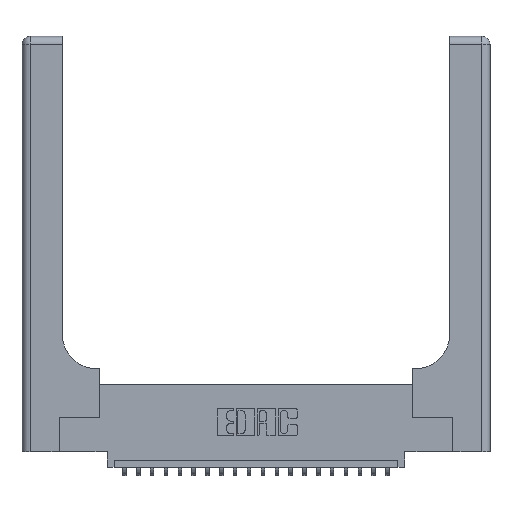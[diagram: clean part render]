
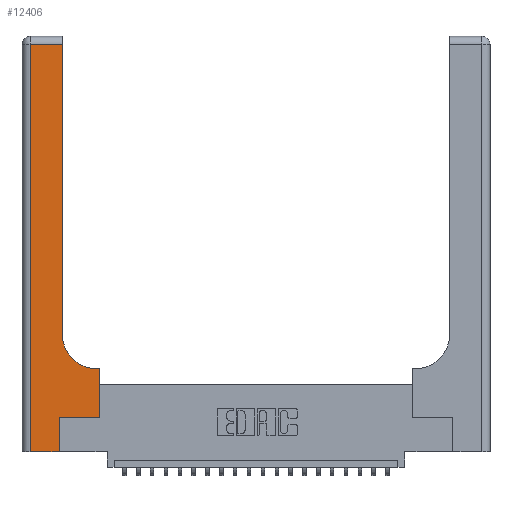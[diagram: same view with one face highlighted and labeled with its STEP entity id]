
A CAD part, top view. The second image highlights one B-rep face of the part: STEP entity #12406.
In plain terms, the highlighted planar face has unit normal (0, 0, 1).
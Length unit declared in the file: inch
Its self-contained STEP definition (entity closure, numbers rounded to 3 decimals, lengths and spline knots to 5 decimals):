
#960 = VECTOR ( 'NONE', #11926, 39.37008 ) ;
#1051 = LINE ( 'NONE', #10312, #22240 ) ;
#1221 = CARTESIAN_POINT ( 'NONE',  ( 0.2915, 0.6, 0.37 ) ) ;
#1324 = DIRECTION ( 'NONE',  ( -1., 0., 0. ) ) ;
#1668 = EDGE_CURVE ( 'NONE', #20339, #4295, #11186, .T. ) ;
#1721 = VERTEX_POINT ( 'NONE', #21738 ) ;
#1817 = CARTESIAN_POINT ( 'NONE',  ( 0.5585, 0.6, 0.37 ) ) ;
#2383 = ORIENTED_EDGE ( 'NONE', *, *, #4557, .T. ) ;
#3017 = VERTEX_POINT ( 'NONE', #7567 ) ;
#3099 = CARTESIAN_POINT ( 'NONE',  ( 0.269, 0., 0.37 ) ) ;
#3658 = EDGE_CURVE ( 'NONE', #6138, #20339, #19414, .T. ) ;
#3685 = ORIENTED_EDGE ( 'NONE', *, *, #5628, .T. ) ;
#3878 = VECTOR ( 'NONE', #6095, 39.37008 ) ;
#4277 = CARTESIAN_POINT ( 'NONE',  ( 0.06, 3., 0.37 ) ) ;
#4295 = VERTEX_POINT ( 'NONE', #11991 ) ;
#4314 = FACE_OUTER_BOUND ( 'NONE', #8168, .T. ) ;
#4333 = DIRECTION ( 'NONE',  ( -1., 0., 0. ) ) ;
#4454 = VECTOR ( 'NONE', #4813, 39.37008 ) ;
#4557 = EDGE_CURVE ( 'NONE', #19125, #6138, #18001, .T. ) ;
#4813 = DIRECTION ( 'NONE',  ( -1., 0., 0. ) ) ;
#5012 = VECTOR ( 'NONE', #18458, 39.37008 ) ;
#5111 = CARTESIAN_POINT ( 'NONE',  ( 0.06, 0., 0.37 ) ) ;
#5488 = CARTESIAN_POINT ( 'NONE',  ( 0.5585, 0.25, 0.37 ) ) ;
#5628 = EDGE_CURVE ( 'NONE', #4295, #3017, #12844, .T. ) ;
#5804 = EDGE_CURVE ( 'NONE', #1721, #12709, #6657, .T. ) ;
#6095 = DIRECTION ( 'NONE',  ( 0., -1., 0. ) ) ;
#6138 = VERTEX_POINT ( 'NONE', #5111 ) ;
#6259 = ORIENTED_EDGE ( 'NONE', *, *, #1668, .T. ) ;
#6657 = LINE ( 'NONE', #9618, #21048 ) ;
#6861 = ORIENTED_EDGE ( 'NONE', *, *, #21499, .T. ) ;
#7369 = VECTOR ( 'NONE', #10957, 39.37008 ) ;
#7567 = CARTESIAN_POINT ( 'NONE',  ( 0.5585, 0.25, 0.37 ) ) ;
#8168 = EDGE_LOOP ( 'NONE', ( #9216, #20726, #2383, #13592, #6259, #3685, #11124, #6861, #22693 ) ) ;
#8589 = DIRECTION ( 'NONE',  ( 1., 0., 0. ) ) ;
#8967 = CARTESIAN_POINT ( 'NONE',  ( 0.5415, 0.6, 0.37 ) ) ;
#9216 = ORIENTED_EDGE ( 'NONE', *, *, #5804, .T. ) ;
#9290 = AXIS2_PLACEMENT_3D ( 'NONE', #13443, #15250, #9794 ) ;
#9618 = CARTESIAN_POINT ( 'NONE',  ( 0.2915, 3., 0.37 ) ) ;
#9794 = DIRECTION ( 'NONE',  ( 1., 0., 0. ) ) ;
#10312 = CARTESIAN_POINT ( 'NONE',  ( 0., 2.94, 0.37 ) ) ;
#10370 = CARTESIAN_POINT ( 'NONE',  ( 0., 3., 0.37 ) ) ;
#10957 = DIRECTION ( 'NONE',  ( 0., 1., 0. ) ) ;
#11124 = ORIENTED_EDGE ( 'NONE', *, *, #13130, .T. ) ;
#11186 = LINE ( 'NONE', #3099, #960 ) ;
#11926 = DIRECTION ( 'NONE',  ( 0., 1., 0. ) ) ;
#11991 = CARTESIAN_POINT ( 'NONE',  ( 0.269, 0.25, 0.37 ) ) ;
#12149 = LINE ( 'NONE', #5488, #7369 ) ;
#12406 = ADVANCED_FACE ( 'NONE', ( #4314 ), #20334, .F. ) ;
#12709 = VERTEX_POINT ( 'NONE', #20183 ) ;
#12844 = LINE ( 'NONE', #17320, #14818 ) ;
#12972 = CARTESIAN_POINT ( 'NONE',  ( 0., 0., 0.37 ) ) ;
#13087 = CIRCLE ( 'NONE', #9290, 0.25 ) ;
#13130 = EDGE_CURVE ( 'NONE', #3017, #19410, #12149, .T. ) ;
#13443 = CARTESIAN_POINT ( 'NONE',  ( 0.5415, 0.85, 0.37 ) ) ;
#13592 = ORIENTED_EDGE ( 'NONE', *, *, #3658, .T. ) ;
#14125 = VERTEX_POINT ( 'NONE', #8967 ) ;
#14818 = VECTOR ( 'NONE', #8589, 39.37008 ) ;
#15250 = DIRECTION ( 'NONE',  ( 0., 0., -1. ) ) ;
#15996 = LINE ( 'NONE', #1221, #4454 ) ;
#17025 = CARTESIAN_POINT ( 'NONE',  ( 0.269, 0., 0.37 ) ) ;
#17320 = CARTESIAN_POINT ( 'NONE',  ( 0.269, 0.25, 0.37 ) ) ;
#18001 = LINE ( 'NONE', #4277, #3878 ) ;
#18458 = DIRECTION ( 'NONE',  ( 1., 0., 0. ) ) ;
#18508 = CARTESIAN_POINT ( 'NONE',  ( 0.06, 2.94, 0.37 ) ) ;
#19103 = DIRECTION ( 'NONE',  ( 0., 0., -1. ) ) ;
#19125 = VERTEX_POINT ( 'NONE', #18508 ) ;
#19410 = VERTEX_POINT ( 'NONE', #1817 ) ;
#19414 = LINE ( 'NONE', #12972, #5012 ) ;
#20173 = DIRECTION ( 'NONE',  ( 0., 1., 0. ) ) ;
#20183 = CARTESIAN_POINT ( 'NONE',  ( 0.2915, 2.94, 0.37 ) ) ;
#20334 = PLANE ( 'NONE',  #21235 ) ;
#20339 = VERTEX_POINT ( 'NONE', #17025 ) ;
#20726 = ORIENTED_EDGE ( 'NONE', *, *, #20926, .T. ) ;
#20926 = EDGE_CURVE ( 'NONE', #12709, #19125, #1051, .T. ) ;
#21048 = VECTOR ( 'NONE', #20173, 39.37008 ) ;
#21235 = AXIS2_PLACEMENT_3D ( 'NONE', #10370, #19103, #4333 ) ;
#21499 = EDGE_CURVE ( 'NONE', #19410, #14125, #15996, .T. ) ;
#21738 = CARTESIAN_POINT ( 'NONE',  ( 0.2915, 0.85, 0.37 ) ) ;
#22240 = VECTOR ( 'NONE', #1324, 39.37008 ) ;
#22693 = ORIENTED_EDGE ( 'NONE', *, *, #22932, .T. ) ;
#22932 = EDGE_CURVE ( 'NONE', #14125, #1721, #13087, .T. ) ;
